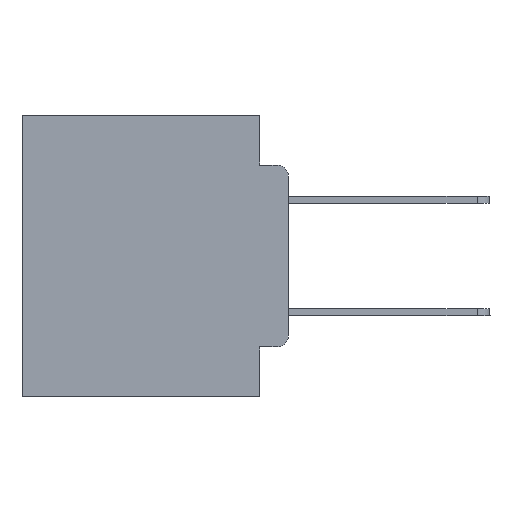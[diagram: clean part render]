
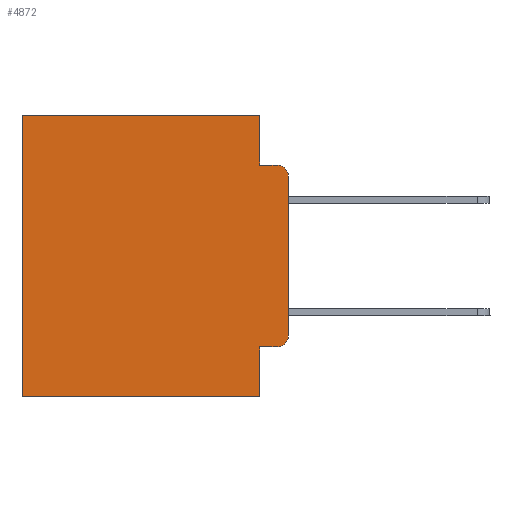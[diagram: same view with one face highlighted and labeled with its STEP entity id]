
A CAD part, left-side view. The second image highlights one B-rep face of the part: STEP entity #4872.
In plain terms, the highlighted planar face has unit normal (-1, 0, 0).
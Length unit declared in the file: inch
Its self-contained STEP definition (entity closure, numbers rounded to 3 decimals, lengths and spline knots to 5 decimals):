
#212 = CIRCLE ( 'NONE', #10137, 0.02 ) ;
#1159 = CARTESIAN_POINT ( 'NONE',  ( 0.298, 0.051, 0. ) ) ;
#1208 = CARTESIAN_POINT ( 'NONE',  ( 0.298, 0.02, -0.3915 ) ) ;
#1609 = CARTESIAN_POINT ( 'NONE',  ( 0.298, 0.051, -0.5 ) ) ;
#1692 = EDGE_CURVE ( 'NONE', #16922, #1697, #25675, .T. ) ;
#1697 = VERTEX_POINT ( 'NONE', #2767 ) ;
#1737 = CARTESIAN_POINT ( 'NONE',  ( 0.298, 0., 0. ) ) ;
#2134 = CARTESIAN_POINT ( 'NONE',  ( 0.298, 0.02, -0.4115 ) ) ;
#2320 = VERTEX_POINT ( 'NONE', #20920 ) ;
#2481 = DIRECTION ( 'NONE',  ( 0., 1., 0. ) ) ;
#2512 = EDGE_CURVE ( 'NONE', #20396, #6781, #4712, .T. ) ;
#2767 = CARTESIAN_POINT ( 'NONE',  ( 0.298, 0.473, -0.5 ) ) ;
#2772 = CARTESIAN_POINT ( 'NONE',  ( 0.298, 0.473, 0. ) ) ;
#2943 = VERTEX_POINT ( 'NONE', #2772 ) ;
#3085 = LINE ( 'NONE', #1159, #7737 ) ;
#3530 = DIRECTION ( 'NONE',  ( 0., 0., -1. ) ) ;
#3662 = EDGE_CURVE ( 'NONE', #20396, #12128, #212, .T. ) ;
#4092 = LINE ( 'NONE', #16329, #18466 ) ;
#4125 = VECTOR ( 'NONE', #2481, 39.37008 ) ;
#4296 = DIRECTION ( 'NONE',  ( 1., 0., 0. ) ) ;
#4419 = ORIENTED_EDGE ( 'NONE', *, *, #6950, .F. ) ;
#4712 = LINE ( 'NONE', #7195, #18926 ) ;
#4717 = CARTESIAN_POINT ( 'NONE',  ( 0.298, 0.02, -0.1085 ) ) ;
#4872 = ADVANCED_FACE ( 'NONE', ( #6369 ), #22851, .F. ) ;
#5236 = CARTESIAN_POINT ( 'NONE',  ( 0.298, 0., -0.3915 ) ) ;
#5843 = EDGE_CURVE ( 'NONE', #24923, #12128, #11355, .T. ) ;
#5864 = CARTESIAN_POINT ( 'NONE',  ( 0.298, 0.473, 0. ) ) ;
#6369 = FACE_OUTER_BOUND ( 'NONE', #25883, .T. ) ;
#6781 = VERTEX_POINT ( 'NONE', #5236 ) ;
#6788 = DIRECTION ( 'NONE',  ( 0., 0., -1. ) ) ;
#6950 = EDGE_CURVE ( 'NONE', #2320, #16922, #11948, .T. ) ;
#7195 = CARTESIAN_POINT ( 'NONE',  ( 0.298, 0., 0. ) ) ;
#7466 = DIRECTION ( 'NONE',  ( 0., 0., -1. ) ) ;
#7564 = DIRECTION ( 'NONE',  ( 0., 0., -1. ) ) ;
#7737 = VECTOR ( 'NONE', #7466, 39.37008 ) ;
#8076 = DIRECTION ( 'NONE',  ( 0., -1., 0. ) ) ;
#9021 = ORIENTED_EDGE ( 'NONE', *, *, #5843, .F. ) ;
#9581 = DIRECTION ( 'NONE',  ( -1., 0., 0. ) ) ;
#9623 = CARTESIAN_POINT ( 'NONE',  ( 0.298, 0.051, 0. ) ) ;
#10094 = DIRECTION ( 'NONE',  ( 0., 1., 0. ) ) ;
#10137 = AXIS2_PLACEMENT_3D ( 'NONE', #4717, #25588, #6788 ) ;
#10476 = VECTOR ( 'NONE', #10094, 39.37008 ) ;
#11160 = DIRECTION ( 'NONE',  ( 0., 0., -1. ) ) ;
#11355 = LINE ( 'NONE', #12889, #18714 ) ;
#11659 = EDGE_CURVE ( 'NONE', #2320, #15509, #4092, .T. ) ;
#11948 = LINE ( 'NONE', #9623, #19660 ) ;
#12128 = VERTEX_POINT ( 'NONE', #25733 ) ;
#12267 = VECTOR ( 'NONE', #3530, 39.37008 ) ;
#12326 = ORIENTED_EDGE ( 'NONE', *, *, #3662, .T. ) ;
#12401 = ORIENTED_EDGE ( 'NONE', *, *, #16987, .T. ) ;
#12670 = DIRECTION ( 'NONE',  ( 0., 0., -1. ) ) ;
#12889 = CARTESIAN_POINT ( 'NONE',  ( 0.298, 0.051, -0.0885 ) ) ;
#13927 = EDGE_CURVE ( 'NONE', #15509, #6781, #25151, .T. ) ;
#14509 = ORIENTED_EDGE ( 'NONE', *, *, #1692, .F. ) ;
#15509 = VERTEX_POINT ( 'NONE', #2134 ) ;
#15823 = CARTESIAN_POINT ( 'NONE',  ( 0.298, 0.051, 0. ) ) ;
#16329 = CARTESIAN_POINT ( 'NONE',  ( 0.298, 0.051, -0.4115 ) ) ;
#16371 = CARTESIAN_POINT ( 'NONE',  ( 0.298, 0., -0.1085 ) ) ;
#16430 = LINE ( 'NONE', #1737, #10476 ) ;
#16451 = ORIENTED_EDGE ( 'NONE', *, *, #13927, .T. ) ;
#16922 = VERTEX_POINT ( 'NONE', #1609 ) ;
#16962 = EDGE_CURVE ( 'NONE', #2943, #1697, #18356, .T. ) ;
#16987 = EDGE_CURVE ( 'NONE', #20973, #2943, #16430, .T. ) ;
#17278 = DIRECTION ( 'NONE',  ( 0., -1., 0. ) ) ;
#17694 = AXIS2_PLACEMENT_3D ( 'NONE', #1208, #9581, #26315 ) ;
#17974 = CARTESIAN_POINT ( 'NONE',  ( 0.298, 0., -0.5 ) ) ;
#18356 = LINE ( 'NONE', #5864, #12267 ) ;
#18466 = VECTOR ( 'NONE', #8076, 39.37008 ) ;
#18714 = VECTOR ( 'NONE', #17278, 39.37008 ) ;
#18857 = CARTESIAN_POINT ( 'NONE',  ( 0.298, 0., 0. ) ) ;
#18926 = VECTOR ( 'NONE', #11160, 39.37008 ) ;
#19311 = ORIENTED_EDGE ( 'NONE', *, *, #2512, .F. ) ;
#19494 = ORIENTED_EDGE ( 'NONE', *, *, #21621, .F. ) ;
#19660 = VECTOR ( 'NONE', #7564, 39.37008 ) ;
#20396 = VERTEX_POINT ( 'NONE', #16371 ) ;
#20426 = CARTESIAN_POINT ( 'NONE',  ( 0.298, 0.051, -0.0885 ) ) ;
#20920 = CARTESIAN_POINT ( 'NONE',  ( 0.298, 0.051, -0.4115 ) ) ;
#20973 = VERTEX_POINT ( 'NONE', #15823 ) ;
#21621 = EDGE_CURVE ( 'NONE', #20973, #24923, #3085, .T. ) ;
#22851 = PLANE ( 'NONE',  #24817 ) ;
#24659 = ORIENTED_EDGE ( 'NONE', *, *, #11659, .T. ) ;
#24817 = AXIS2_PLACEMENT_3D ( 'NONE', #18857, #4296, #12670 ) ;
#24923 = VERTEX_POINT ( 'NONE', #20426 ) ;
#25151 = CIRCLE ( 'NONE', #17694, 0.02 ) ;
#25588 = DIRECTION ( 'NONE',  ( -1., 0., 0. ) ) ;
#25675 = LINE ( 'NONE', #17974, #4125 ) ;
#25733 = CARTESIAN_POINT ( 'NONE',  ( 0.298, 0.02, -0.0885 ) ) ;
#25883 = EDGE_LOOP ( 'NONE', ( #19311, #12326, #9021, #19494, #12401, #26410, #14509, #4419, #24659, #16451 ) ) ;
#26315 = DIRECTION ( 'NONE',  ( 0., 0., -1. ) ) ;
#26410 = ORIENTED_EDGE ( 'NONE', *, *, #16962, .T. ) ;
